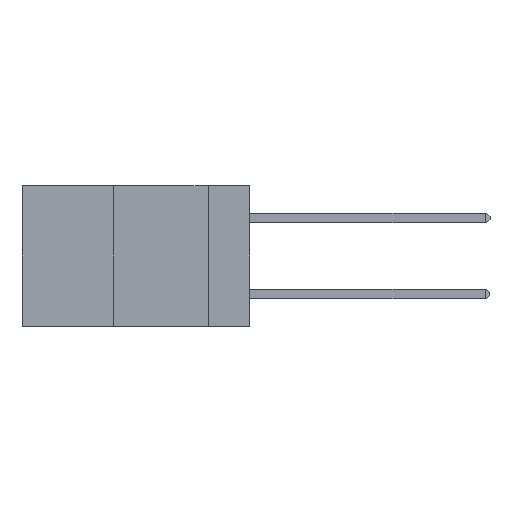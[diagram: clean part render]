
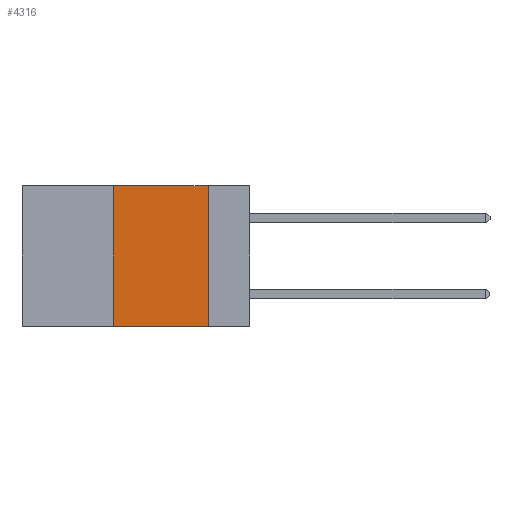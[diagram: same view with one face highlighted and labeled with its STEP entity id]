
A CAD part, left-side view. The second image highlights one B-rep face of the part: STEP entity #4316.
In plain terms, the highlighted planar face has unit normal (-1, 0, 0).
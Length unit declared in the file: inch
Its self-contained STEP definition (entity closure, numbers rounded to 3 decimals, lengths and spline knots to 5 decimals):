
#143 = VERTEX_POINT ( 'NONE', #7886 ) ;
#1490 = EDGE_CURVE ( 'NONE', #6440, #143, #12006, .T. ) ;
#1847 = EDGE_LOOP ( 'NONE', ( #10116, #7977, #2056, #3438 ) ) ;
#2056 = ORIENTED_EDGE ( 'NONE', *, *, #1490, .F. ) ;
#2186 = LINE ( 'NONE', #3002, #5132 ) ;
#2325 = CARTESIAN_POINT ( 'NONE',  ( 0., 0.11, 0. ) ) ;
#2866 = DIRECTION ( 'NONE',  ( 0., 0., -1. ) ) ;
#3002 = CARTESIAN_POINT ( 'NONE',  ( 0., 0.6, -0.37 ) ) ;
#3121 = DIRECTION ( 'NONE',  ( 1., 0., 0. ) ) ;
#3214 = CARTESIAN_POINT ( 'NONE',  ( 0., 0.6, 0. ) ) ;
#3233 = PLANE ( 'NONE',  #5292 ) ;
#3438 = ORIENTED_EDGE ( 'NONE', *, *, #14757, .T. ) ;
#4316 = ADVANCED_FACE ( 'NONE', ( #4714 ), #3233, .F. ) ;
#4357 = CARTESIAN_POINT ( 'NONE',  ( 0., 0.6, 0. ) ) ;
#4714 = FACE_OUTER_BOUND ( 'NONE', #1847, .T. ) ;
#4967 = VECTOR ( 'NONE', #9307, 39.37008 ) ;
#5132 = VECTOR ( 'NONE', #11730, 39.37008 ) ;
#5292 = AXIS2_PLACEMENT_3D ( 'NONE', #3214, #3121, #2866 ) ;
#5665 = DIRECTION ( 'NONE',  ( 0., -1., 0. ) ) ;
#6440 = VERTEX_POINT ( 'NONE', #7671 ) ;
#7379 = CARTESIAN_POINT ( 'NONE',  ( 0., 0.11, 0. ) ) ;
#7671 = CARTESIAN_POINT ( 'NONE',  ( 0., 0.36, -0.37 ) ) ;
#7886 = CARTESIAN_POINT ( 'NONE',  ( 0., 0.36, 0. ) ) ;
#7957 = EDGE_CURVE ( 'NONE', #143, #9094, #12776, .T. ) ;
#7977 = ORIENTED_EDGE ( 'NONE', *, *, #7957, .F. ) ;
#9094 = VERTEX_POINT ( 'NONE', #7379 ) ;
#9141 = VECTOR ( 'NONE', #5665, 39.37008 ) ;
#9307 = DIRECTION ( 'NONE',  ( 0., 0., 1. ) ) ;
#9372 = CARTESIAN_POINT ( 'NONE',  ( 0., 0.36, 0. ) ) ;
#9665 = VECTOR ( 'NONE', #12320, 39.37008 ) ;
#10116 = ORIENTED_EDGE ( 'NONE', *, *, #15070, .F. ) ;
#11730 = DIRECTION ( 'NONE',  ( 0., -1., 0. ) ) ;
#12006 = LINE ( 'NONE', #9372, #4967 ) ;
#12320 = DIRECTION ( 'NONE',  ( 0., 0., -1. ) ) ;
#12776 = LINE ( 'NONE', #4357, #9141 ) ;
#14517 = VERTEX_POINT ( 'NONE', #15697 ) ;
#14757 = EDGE_CURVE ( 'NONE', #6440, #14517, #2186, .T. ) ;
#15070 = EDGE_CURVE ( 'NONE', #9094, #14517, #15656, .T. ) ;
#15656 = LINE ( 'NONE', #2325, #9665 ) ;
#15697 = CARTESIAN_POINT ( 'NONE',  ( 0., 0.11, -0.37 ) ) ;
